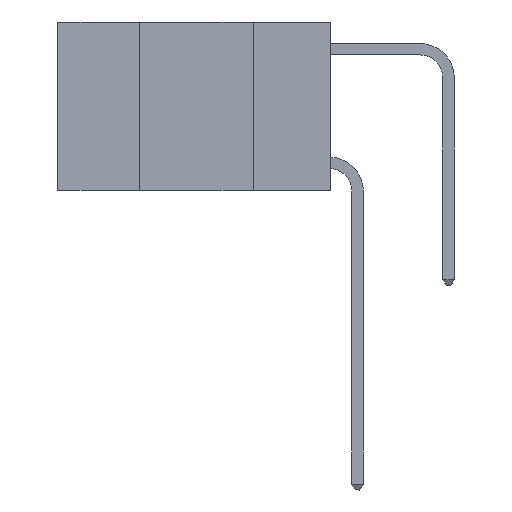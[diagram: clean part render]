
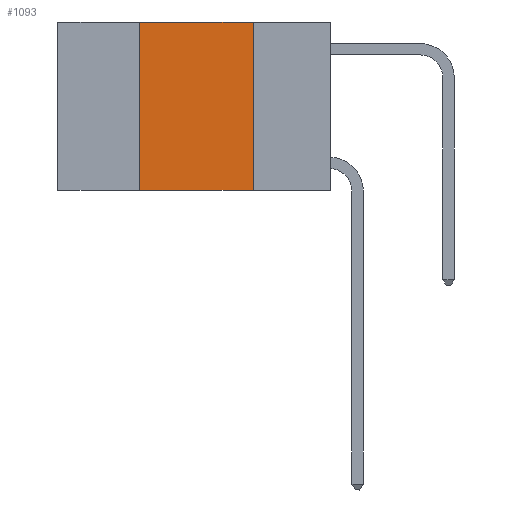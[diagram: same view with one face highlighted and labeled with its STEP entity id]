
A CAD part, left-side view. The second image highlights one B-rep face of the part: STEP entity #1093.
In plain terms, the highlighted planar face has unit normal (-1, 0, 0).
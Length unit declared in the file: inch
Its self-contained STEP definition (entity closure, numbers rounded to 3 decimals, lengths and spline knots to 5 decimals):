
#694 = ORIENTED_EDGE ( 'NONE', *, *, #9324, .T. ) ;
#1093 = ADVANCED_FACE ( 'NONE', ( #7339 ), #6908, .F. ) ;
#2065 = DIRECTION ( 'NONE',  ( 0., 0., -1. ) ) ;
#3435 = CARTESIAN_POINT ( 'NONE',  ( 0., 0.17, 0. ) ) ;
#4014 = EDGE_CURVE ( 'NONE', #5014, #4614, #10577, .T. ) ;
#4614 = VERTEX_POINT ( 'NONE', #12644 ) ;
#5014 = VERTEX_POINT ( 'NONE', #3435 ) ;
#5016 = VECTOR ( 'NONE', #8807, 39.37008 ) ;
#5099 = ORIENTED_EDGE ( 'NONE', *, *, #6343, .F. ) ;
#5202 = DIRECTION ( 'NONE',  ( 0., -1., 0. ) ) ;
#5210 = VERTEX_POINT ( 'NONE', #12246 ) ;
#5602 = DIRECTION ( 'NONE',  ( 0., 0., 1. ) ) ;
#6241 = DIRECTION ( 'NONE',  ( 0., 0., -1. ) ) ;
#6324 = DIRECTION ( 'NONE',  ( 1., 0., 0. ) ) ;
#6343 = EDGE_CURVE ( 'NONE', #10852, #5014, #10628, .T. ) ;
#6698 = CARTESIAN_POINT ( 'NONE',  ( 0., 0.42, 0. ) ) ;
#6738 = CARTESIAN_POINT ( 'NONE',  ( 0., 0.6, 0. ) ) ;
#6908 = PLANE ( 'NONE',  #12674 ) ;
#7339 = FACE_OUTER_BOUND ( 'NONE', #8622, .T. ) ;
#7395 = VECTOR ( 'NONE', #2065, 39.37008 ) ;
#7821 = VECTOR ( 'NONE', #5602, 39.37008 ) ;
#8622 = EDGE_LOOP ( 'NONE', ( #11893, #5099, #11199, #694 ) ) ;
#8807 = DIRECTION ( 'NONE',  ( 0., -1., 0. ) ) ;
#9324 = EDGE_CURVE ( 'NONE', #5210, #4614, #10730, .T. ) ;
#10577 = LINE ( 'NONE', #10829, #7395 ) ;
#10628 = LINE ( 'NONE', #12469, #12812 ) ;
#10730 = LINE ( 'NONE', #10949, #5016 ) ;
#10829 = CARTESIAN_POINT ( 'NONE',  ( 0., 0.17, 0. ) ) ;
#10852 = VERTEX_POINT ( 'NONE', #11258 ) ;
#10949 = CARTESIAN_POINT ( 'NONE',  ( 0., 0.6, -0.37 ) ) ;
#11199 = ORIENTED_EDGE ( 'NONE', *, *, #11489, .F. ) ;
#11258 = CARTESIAN_POINT ( 'NONE',  ( 0., 0.42, 0. ) ) ;
#11489 = EDGE_CURVE ( 'NONE', #5210, #10852, #13521, .T. ) ;
#11893 = ORIENTED_EDGE ( 'NONE', *, *, #4014, .F. ) ;
#12246 = CARTESIAN_POINT ( 'NONE',  ( 0., 0.42, -0.37 ) ) ;
#12469 = CARTESIAN_POINT ( 'NONE',  ( 0., 0.6, 0. ) ) ;
#12644 = CARTESIAN_POINT ( 'NONE',  ( 0., 0.17, -0.37 ) ) ;
#12674 = AXIS2_PLACEMENT_3D ( 'NONE', #6738, #6324, #6241 ) ;
#12812 = VECTOR ( 'NONE', #5202, 39.37008 ) ;
#13521 = LINE ( 'NONE', #6698, #7821 ) ;
